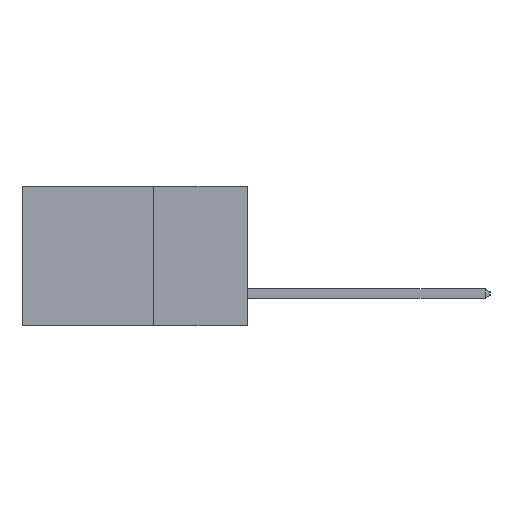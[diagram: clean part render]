
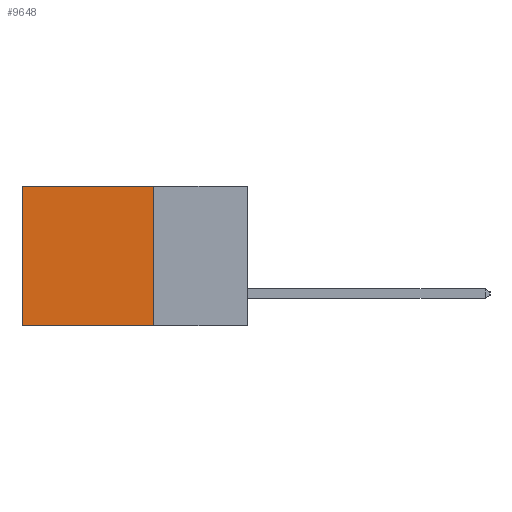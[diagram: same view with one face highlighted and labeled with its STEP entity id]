
A CAD part, left-side view. The second image highlights one B-rep face of the part: STEP entity #9648.
In plain terms, the highlighted planar face has unit normal (-1, 0, 0).
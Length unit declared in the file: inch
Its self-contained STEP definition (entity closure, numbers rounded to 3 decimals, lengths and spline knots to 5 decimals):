
#10 = CARTESIAN_POINT ( 'NONE',  ( 0.298, 0.6, 0. ) ) ;
#1362 = ORIENTED_EDGE ( 'NONE', *, *, #12700, .T. ) ;
#1748 = DIRECTION ( 'NONE',  ( 1., 0., 0. ) ) ;
#2575 = LINE ( 'NONE', #10, #16894 ) ;
#3257 = LINE ( 'NONE', #4807, #13034 ) ;
#3398 = ORIENTED_EDGE ( 'NONE', *, *, #23230, .T. ) ;
#3613 = ORIENTED_EDGE ( 'NONE', *, *, #4105, .F. ) ;
#3653 = LINE ( 'NONE', #20600, #18487 ) ;
#3984 = VECTOR ( 'NONE', #9588, 39.37008 ) ;
#4006 = EDGE_LOOP ( 'NONE', ( #1362, #3613, #7084, #3398 ) ) ;
#4105 = EDGE_CURVE ( 'NONE', #13147, #11594, #3653, .T. ) ;
#4211 = DIRECTION ( 'NONE',  ( 0., 1., 0. ) ) ;
#4807 = CARTESIAN_POINT ( 'NONE',  ( 0.298, 0.25, 0. ) ) ;
#5323 = CARTESIAN_POINT ( 'NONE',  ( 0.298, 0.6, 0. ) ) ;
#6214 = CARTESIAN_POINT ( 'NONE',  ( 0.298, 0.6, -0.37 ) ) ;
#7084 = ORIENTED_EDGE ( 'NONE', *, *, #9010, .F. ) ;
#7458 = VERTEX_POINT ( 'NONE', #14820 ) ;
#9010 = EDGE_CURVE ( 'NONE', #7458, #13147, #14349, .T. ) ;
#9588 = DIRECTION ( 'NONE',  ( 0., 0., -1. ) ) ;
#9648 = ADVANCED_FACE ( 'NONE', ( #10711 ), #11564, .F. ) ;
#10711 = FACE_OUTER_BOUND ( 'NONE', #4006, .T. ) ;
#11564 = PLANE ( 'NONE',  #12152 ) ;
#11594 = VERTEX_POINT ( 'NONE', #6214 ) ;
#12152 = AXIS2_PLACEMENT_3D ( 'NONE', #24927, #1748, #15454 ) ;
#12700 = EDGE_CURVE ( 'NONE', #20370, #11594, #2575, .T. ) ;
#13034 = VECTOR ( 'NONE', #24118, 39.37008 ) ;
#13147 = VERTEX_POINT ( 'NONE', #22820 ) ;
#14349 = LINE ( 'NONE', #15323, #3984 ) ;
#14820 = CARTESIAN_POINT ( 'NONE',  ( 0.298, 0.25, 0. ) ) ;
#15323 = CARTESIAN_POINT ( 'NONE',  ( 0.298, 0.25, 0. ) ) ;
#15454 = DIRECTION ( 'NONE',  ( 0., 0., -1. ) ) ;
#16894 = VECTOR ( 'NONE', #21411, 39.37008 ) ;
#18487 = VECTOR ( 'NONE', #4211, 39.37008 ) ;
#20370 = VERTEX_POINT ( 'NONE', #5323 ) ;
#20600 = CARTESIAN_POINT ( 'NONE',  ( 0.298, 0.25, -0.37 ) ) ;
#21411 = DIRECTION ( 'NONE',  ( 0., 0., -1. ) ) ;
#22820 = CARTESIAN_POINT ( 'NONE',  ( 0.298, 0.25, -0.37 ) ) ;
#23230 = EDGE_CURVE ( 'NONE', #7458, #20370, #3257, .T. ) ;
#24118 = DIRECTION ( 'NONE',  ( 0., 1., 0. ) ) ;
#24927 = CARTESIAN_POINT ( 'NONE',  ( 0.298, 0.25, 0. ) ) ;
